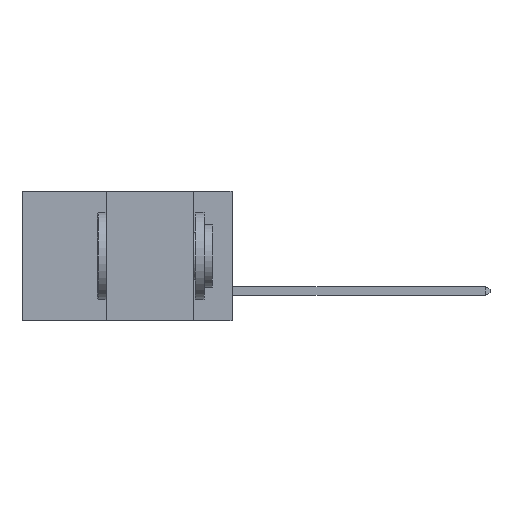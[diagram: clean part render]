
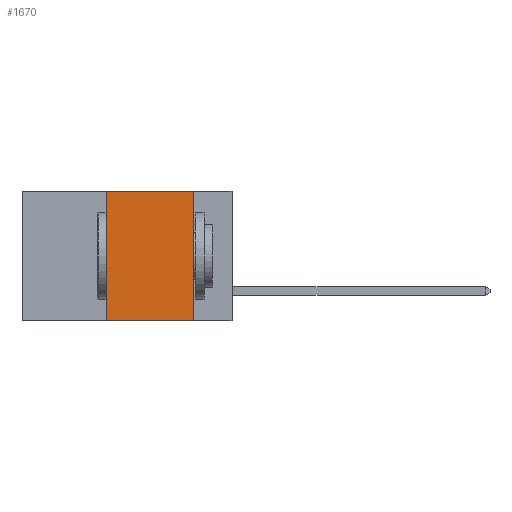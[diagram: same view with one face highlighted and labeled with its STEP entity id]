
A CAD part, left-side view. The second image highlights one B-rep face of the part: STEP entity #1670.
In plain terms, the highlighted planar face has unit normal (-1, 0, 0).
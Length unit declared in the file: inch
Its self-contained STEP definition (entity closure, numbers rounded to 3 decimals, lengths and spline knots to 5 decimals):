
#994 = CARTESIAN_POINT ( 'NONE',  ( 0., 0.36, 0. ) ) ;
#1130 = CARTESIAN_POINT ( 'NONE',  ( 0., 0.36, -0.37 ) ) ;
#1670 = ADVANCED_FACE ( 'NONE', ( #20484 ), #32016, .F. ) ;
#2245 = VECTOR ( 'NONE', #27069, 39.37008 ) ;
#3337 = ORIENTED_EDGE ( 'NONE', *, *, #13407, .T. ) ;
#6247 = LINE ( 'NONE', #19053, #19210 ) ;
#6257 = VERTEX_POINT ( 'NONE', #30580 ) ;
#7085 = VERTEX_POINT ( 'NONE', #994 ) ;
#7324 = EDGE_LOOP ( 'NONE', ( #31340, #25722, #31584, #3337 ) ) ;
#8909 = CARTESIAN_POINT ( 'NONE',  ( 0., 0.36, 0. ) ) ;
#9601 = DIRECTION ( 'NONE',  ( 0., 0., -1. ) ) ;
#9641 = DIRECTION ( 'NONE',  ( 1., 0., 0. ) ) ;
#10075 = DIRECTION ( 'NONE',  ( 0., -1., 0. ) ) ;
#11548 = DIRECTION ( 'NONE',  ( 0., 0., 1. ) ) ;
#12291 = EDGE_CURVE ( 'NONE', #16555, #7085, #18981, .T. ) ;
#12559 = CARTESIAN_POINT ( 'NONE',  ( 0., 0.6, 0. ) ) ;
#13015 = LINE ( 'NONE', #12559, #24173 ) ;
#13407 = EDGE_CURVE ( 'NONE', #16555, #24133, #29501, .T. ) ;
#14640 = EDGE_CURVE ( 'NONE', #6257, #24133, #6247, .T. ) ;
#16555 = VERTEX_POINT ( 'NONE', #1130 ) ;
#18981 = LINE ( 'NONE', #8909, #31530 ) ;
#19053 = CARTESIAN_POINT ( 'NONE',  ( 0., 0.11, 0. ) ) ;
#19210 = VECTOR ( 'NONE', #21601, 39.37008 ) ;
#19466 = CARTESIAN_POINT ( 'NONE',  ( 0., 0.6, -0.37 ) ) ;
#20484 = FACE_OUTER_BOUND ( 'NONE', #7324, .T. ) ;
#21601 = DIRECTION ( 'NONE',  ( 0., 0., -1. ) ) ;
#22147 = CARTESIAN_POINT ( 'NONE',  ( 0., 0.11, -0.37 ) ) ;
#24133 = VERTEX_POINT ( 'NONE', #22147 ) ;
#24173 = VECTOR ( 'NONE', #10075, 39.37008 ) ;
#25722 = ORIENTED_EDGE ( 'NONE', *, *, #32553, .F. ) ;
#27069 = DIRECTION ( 'NONE',  ( 0., -1., 0. ) ) ;
#29501 = LINE ( 'NONE', #19466, #2245 ) ;
#30580 = CARTESIAN_POINT ( 'NONE',  ( 0., 0.11, 0. ) ) ;
#31340 = ORIENTED_EDGE ( 'NONE', *, *, #14640, .F. ) ;
#31341 = CARTESIAN_POINT ( 'NONE',  ( 0., 0.6, 0. ) ) ;
#31530 = VECTOR ( 'NONE', #11548, 39.37008 ) ;
#31584 = ORIENTED_EDGE ( 'NONE', *, *, #12291, .F. ) ;
#32016 = PLANE ( 'NONE',  #32371 ) ;
#32371 = AXIS2_PLACEMENT_3D ( 'NONE', #31341, #9641, #9601 ) ;
#32553 = EDGE_CURVE ( 'NONE', #7085, #6257, #13015, .T. ) ;
